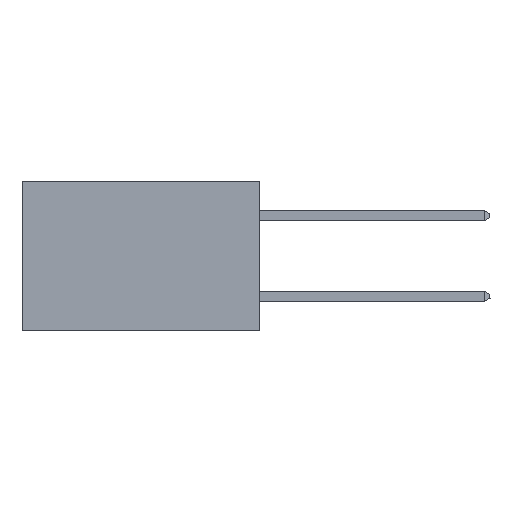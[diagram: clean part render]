
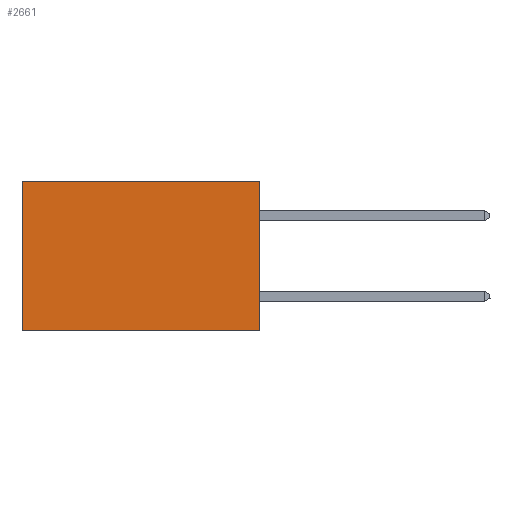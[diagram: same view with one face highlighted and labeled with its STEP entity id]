
A CAD part, left-side view. The second image highlights one B-rep face of the part: STEP entity #2661.
In plain terms, the highlighted planar face has unit normal (-1, 0, 0).
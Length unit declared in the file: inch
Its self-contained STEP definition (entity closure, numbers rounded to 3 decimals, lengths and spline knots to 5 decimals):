
#799 = ORIENTED_EDGE ( 'NONE', *, *, #9105, .F. ) ;
#1007 = PLANE ( 'NONE',  #21306 ) ;
#2046 = VERTEX_POINT ( 'NONE', #15416 ) ;
#2661 = ADVANCED_FACE ( 'NONE', ( #11926 ), #1007, .F. ) ;
#3016 = VERTEX_POINT ( 'NONE', #8002 ) ;
#3562 = EDGE_CURVE ( 'NONE', #4874, #9808, #7709, .T. ) ;
#4874 = VERTEX_POINT ( 'NONE', #21855 ) ;
#5856 = ORIENTED_EDGE ( 'NONE', *, *, #7030, .F. ) ;
#5870 = EDGE_CURVE ( 'NONE', #9808, #2046, #13649, .T. ) ;
#6714 = CARTESIAN_POINT ( 'NONE',  ( 0.277, 0., 0. ) ) ;
#7030 = EDGE_CURVE ( 'NONE', #4874, #3016, #8831, .T. ) ;
#7709 = LINE ( 'NONE', #6714, #16180 ) ;
#7800 = DIRECTION ( 'NONE',  ( 1., 0., 0. ) ) ;
#7967 = DIRECTION ( 'NONE',  ( 0., 0., -1. ) ) ;
#8002 = CARTESIAN_POINT ( 'NONE',  ( 0.277, 0., -0.37 ) ) ;
#8736 = CARTESIAN_POINT ( 'NONE',  ( 0.277, 0., -0.37 ) ) ;
#8831 = LINE ( 'NONE', #9663, #9362 ) ;
#8848 = DIRECTION ( 'NONE',  ( 0., 1., 0. ) ) ;
#9105 = EDGE_CURVE ( 'NONE', #3016, #2046, #21365, .T. ) ;
#9362 = VECTOR ( 'NONE', #9643, 39.37008 ) ;
#9643 = DIRECTION ( 'NONE',  ( 0., 0., -1. ) ) ;
#9663 = CARTESIAN_POINT ( 'NONE',  ( 0.277, 0., -0.37 ) ) ;
#9808 = VERTEX_POINT ( 'NONE', #14886 ) ;
#11926 = FACE_OUTER_BOUND ( 'NONE', #15564, .T. ) ;
#12944 = ORIENTED_EDGE ( 'NONE', *, *, #5870, .T. ) ;
#13357 = DIRECTION ( 'NONE',  ( 0., 1., 0. ) ) ;
#13649 = LINE ( 'NONE', #20464, #21014 ) ;
#14180 = ORIENTED_EDGE ( 'NONE', *, *, #3562, .T. ) ;
#14886 = CARTESIAN_POINT ( 'NONE',  ( 0.277, 0.59, 0. ) ) ;
#15416 = CARTESIAN_POINT ( 'NONE',  ( 0.277, 0.59, -0.37 ) ) ;
#15564 = EDGE_LOOP ( 'NONE', ( #12944, #799, #5856, #14180 ) ) ;
#16180 = VECTOR ( 'NONE', #13357, 39.37008 ) ;
#16951 = VECTOR ( 'NONE', #8848, 39.37008 ) ;
#20419 = DIRECTION ( 'NONE',  ( 0., 0., -1. ) ) ;
#20464 = CARTESIAN_POINT ( 'NONE',  ( 0.277, 0.59, -0.37 ) ) ;
#21014 = VECTOR ( 'NONE', #20419, 39.37008 ) ;
#21306 = AXIS2_PLACEMENT_3D ( 'NONE', #21805, #7800, #7967 ) ;
#21365 = LINE ( 'NONE', #8736, #16951 ) ;
#21805 = CARTESIAN_POINT ( 'NONE',  ( 0.277, 0., -0.37 ) ) ;
#21855 = CARTESIAN_POINT ( 'NONE',  ( 0.277, 0., 0. ) ) ;
